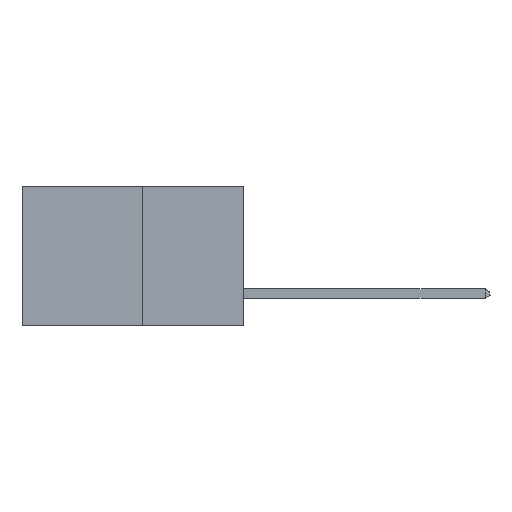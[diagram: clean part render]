
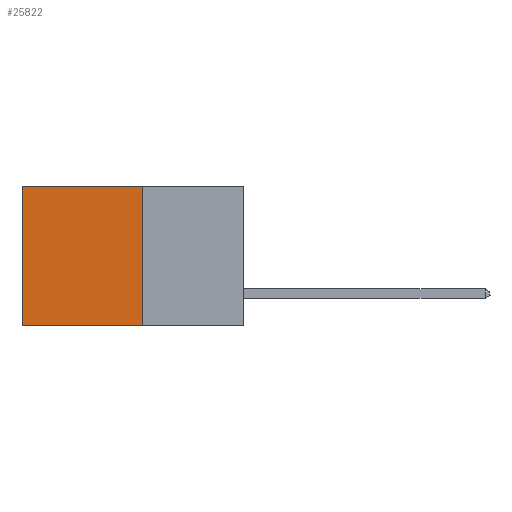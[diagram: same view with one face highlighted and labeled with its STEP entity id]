
A CAD part, left-side view. The second image highlights one B-rep face of the part: STEP entity #25822.
In plain terms, the highlighted planar face has unit normal (-1, 0, 0).
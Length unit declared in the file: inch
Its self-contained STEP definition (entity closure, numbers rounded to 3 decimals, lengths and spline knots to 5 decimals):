
#668 = AXIS2_PLACEMENT_3D ( 'NONE', #16583, #2248, #16674 ) ;
#1258 = VECTOR ( 'NONE', #22744, 39.37008 ) ;
#1777 = CARTESIAN_POINT ( 'NONE',  ( 0.277, 0.59, -0.37 ) ) ;
#2248 = DIRECTION ( 'NONE',  ( 1., 0., 0. ) ) ;
#3120 = VECTOR ( 'NONE', #19904, 39.37008 ) ;
#3337 = CARTESIAN_POINT ( 'NONE',  ( 0.277, 0.27, 0. ) ) ;
#3827 = DIRECTION ( 'NONE',  ( 0., 0., -1. ) ) ;
#4134 = LINE ( 'NONE', #3337, #9627 ) ;
#6485 = CARTESIAN_POINT ( 'NONE',  ( 0.277, 0.27, -0.37 ) ) ;
#6652 = CARTESIAN_POINT ( 'NONE',  ( 0.277, 0.59, 0. ) ) ;
#7578 = ORIENTED_EDGE ( 'NONE', *, *, #12620, .F. ) ;
#7668 = CARTESIAN_POINT ( 'NONE',  ( 0.277, 0.27, -0.37 ) ) ;
#8304 = PLANE ( 'NONE',  #668 ) ;
#9540 = FACE_OUTER_BOUND ( 'NONE', #13257, .T. ) ;
#9627 = VECTOR ( 'NONE', #17726, 39.37008 ) ;
#11926 = ORIENTED_EDGE ( 'NONE', *, *, #18946, .F. ) ;
#12185 = LINE ( 'NONE', #6485, #1258 ) ;
#12620 = EDGE_CURVE ( 'NONE', #22566, #16337, #12185, .T. ) ;
#13055 = ORIENTED_EDGE ( 'NONE', *, *, #13692, .T. ) ;
#13257 = EDGE_LOOP ( 'NONE', ( #13055, #7578, #11926, #22247 ) ) ;
#13405 = CARTESIAN_POINT ( 'NONE',  ( 0.277, 0.59, -0.37 ) ) ;
#13692 = EDGE_CURVE ( 'NONE', #18651, #16337, #20664, .T. ) ;
#15152 = CARTESIAN_POINT ( 'NONE',  ( 0.277, 0.27, -0.37 ) ) ;
#16297 = CARTESIAN_POINT ( 'NONE',  ( 0.277, 0.27, 0. ) ) ;
#16337 = VERTEX_POINT ( 'NONE', #13405 ) ;
#16583 = CARTESIAN_POINT ( 'NONE',  ( 0.277, 0.27, -0.37 ) ) ;
#16674 = DIRECTION ( 'NONE',  ( 0., 0., -1. ) ) ;
#17726 = DIRECTION ( 'NONE',  ( 0., 1., 0. ) ) ;
#18235 = EDGE_CURVE ( 'NONE', #23492, #18651, #4134, .T. ) ;
#18651 = VERTEX_POINT ( 'NONE', #6652 ) ;
#18946 = EDGE_CURVE ( 'NONE', #23492, #22566, #24074, .T. ) ;
#19423 = VECTOR ( 'NONE', #3827, 39.37008 ) ;
#19904 = DIRECTION ( 'NONE',  ( 0., 0., -1. ) ) ;
#20664 = LINE ( 'NONE', #1777, #19423 ) ;
#22247 = ORIENTED_EDGE ( 'NONE', *, *, #18235, .T. ) ;
#22566 = VERTEX_POINT ( 'NONE', #15152 ) ;
#22744 = DIRECTION ( 'NONE',  ( 0., 1., 0. ) ) ;
#23492 = VERTEX_POINT ( 'NONE', #16297 ) ;
#24074 = LINE ( 'NONE', #7668, #3120 ) ;
#25822 = ADVANCED_FACE ( 'NONE', ( #9540 ), #8304, .F. ) ;
